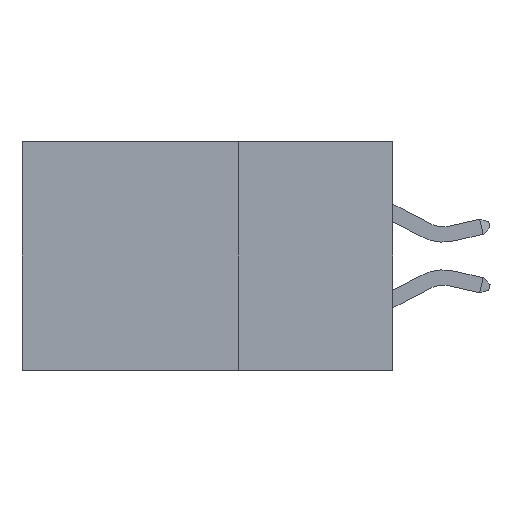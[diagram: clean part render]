
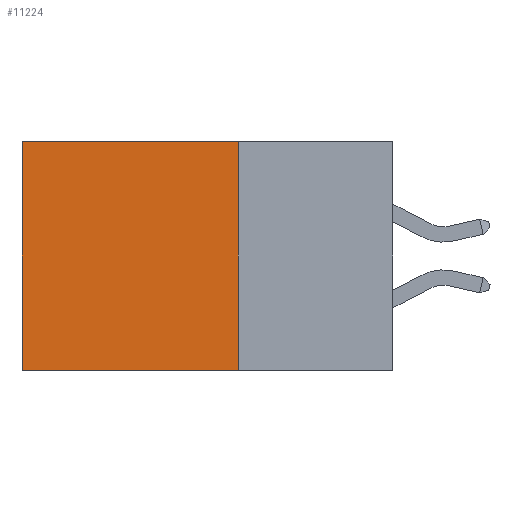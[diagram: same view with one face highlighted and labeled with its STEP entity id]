
A CAD part, left-side view. The second image highlights one B-rep face of the part: STEP entity #11224.
In plain terms, the highlighted planar face has unit normal (-1, 0, 0).
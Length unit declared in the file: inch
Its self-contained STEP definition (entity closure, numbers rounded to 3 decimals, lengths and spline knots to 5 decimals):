
#111 = DIRECTION ( 'NONE',  ( 0., 0., -1. ) ) ;
#1223 = AXIS2_PLACEMENT_3D ( 'NONE', #16973, #19144, #111 ) ;
#1269 = EDGE_CURVE ( 'NONE', #26809, #6972, #16242, .T. ) ;
#1496 = CARTESIAN_POINT ( 'NONE',  ( 0.2875, 0.6, -0.37 ) ) ;
#1774 = CARTESIAN_POINT ( 'NONE',  ( 0.2875, 0.6, 0. ) ) ;
#4140 = FACE_OUTER_BOUND ( 'NONE', #13379, .T. ) ;
#5328 = CARTESIAN_POINT ( 'NONE',  ( 0.2875, 0.25, 0. ) ) ;
#6453 = CARTESIAN_POINT ( 'NONE',  ( 0.2875, 0.6, 0. ) ) ;
#6972 = VERTEX_POINT ( 'NONE', #1496 ) ;
#7301 = LINE ( 'NONE', #8421, #8400 ) ;
#7976 = DIRECTION ( 'NONE',  ( 0., 0., -1. ) ) ;
#8400 = VECTOR ( 'NONE', #29554, 39.37008 ) ;
#8421 = CARTESIAN_POINT ( 'NONE',  ( 0.2875, 0.25, -0.37 ) ) ;
#8533 = VECTOR ( 'NONE', #15518, 39.37008 ) ;
#11224 = ADVANCED_FACE ( 'NONE', ( #4140 ), #23989, .F. ) ;
#12806 = VECTOR ( 'NONE', #7976, 39.37008 ) ;
#13178 = CARTESIAN_POINT ( 'NONE',  ( 0.2875, 0.25, 0. ) ) ;
#13379 = EDGE_LOOP ( 'NONE', ( #29869, #24624, #23954, #26668 ) ) ;
#14227 = EDGE_CURVE ( 'NONE', #26188, #22735, #16507, .T. ) ;
#15518 = DIRECTION ( 'NONE',  ( 0., 1., 0. ) ) ;
#15940 = EDGE_CURVE ( 'NONE', #26188, #26809, #18853, .T. ) ;
#16242 = LINE ( 'NONE', #1774, #26151 ) ;
#16507 = LINE ( 'NONE', #5328, #12806 ) ;
#16973 = CARTESIAN_POINT ( 'NONE',  ( 0.2875, 0.25, 0. ) ) ;
#18853 = LINE ( 'NONE', #13178, #8533 ) ;
#19144 = DIRECTION ( 'NONE',  ( 1., 0., 0. ) ) ;
#20172 = CARTESIAN_POINT ( 'NONE',  ( 0.2875, 0.25, -0.37 ) ) ;
#20625 = CARTESIAN_POINT ( 'NONE',  ( 0.2875, 0.25, 0. ) ) ;
#22735 = VERTEX_POINT ( 'NONE', #20172 ) ;
#22749 = EDGE_CURVE ( 'NONE', #22735, #6972, #7301, .T. ) ;
#23954 = ORIENTED_EDGE ( 'NONE', *, *, #14227, .F. ) ;
#23989 = PLANE ( 'NONE',  #1223 ) ;
#24624 = ORIENTED_EDGE ( 'NONE', *, *, #22749, .F. ) ;
#26151 = VECTOR ( 'NONE', #29991, 39.37008 ) ;
#26188 = VERTEX_POINT ( 'NONE', #20625 ) ;
#26668 = ORIENTED_EDGE ( 'NONE', *, *, #15940, .T. ) ;
#26809 = VERTEX_POINT ( 'NONE', #6453 ) ;
#29554 = DIRECTION ( 'NONE',  ( 0., 1., 0. ) ) ;
#29869 = ORIENTED_EDGE ( 'NONE', *, *, #1269, .T. ) ;
#29991 = DIRECTION ( 'NONE',  ( 0., 0., -1. ) ) ;
